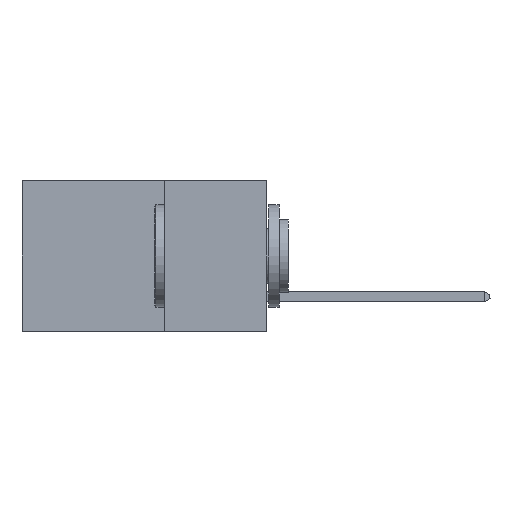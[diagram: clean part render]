
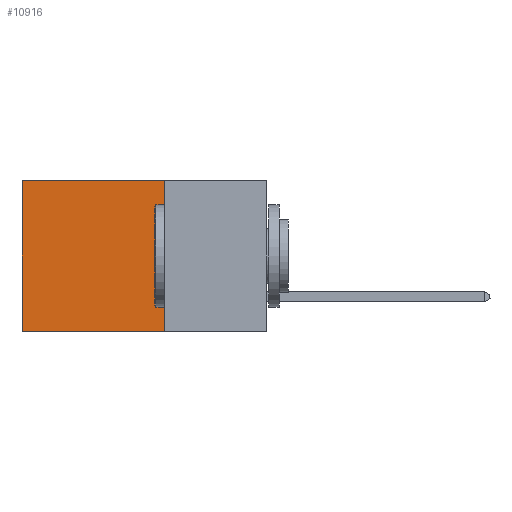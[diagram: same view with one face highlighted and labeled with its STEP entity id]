
A CAD part, left-side view. The second image highlights one B-rep face of the part: STEP entity #10916.
In plain terms, the highlighted planar face has unit normal (-1, 0, 0).
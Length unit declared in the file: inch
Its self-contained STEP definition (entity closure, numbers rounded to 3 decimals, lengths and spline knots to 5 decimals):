
#178 = CARTESIAN_POINT ( 'NONE',  ( 0.2875, 0.25, -0.37 ) ) ;
#617 = CARTESIAN_POINT ( 'NONE',  ( 0.2875, 0.25, 0. ) ) ;
#843 = VERTEX_POINT ( 'NONE', #9537 ) ;
#1072 = VECTOR ( 'NONE', #3567, 39.37008 ) ;
#1185 = DIRECTION ( 'NONE',  ( 0., 1., 0. ) ) ;
#1493 = DIRECTION ( 'NONE',  ( 0., 1., 0. ) ) ;
#1998 = EDGE_CURVE ( 'NONE', #10642, #5314, #9205, .T. ) ;
#2321 = CARTESIAN_POINT ( 'NONE',  ( 0.2875, 0.25, 0. ) ) ;
#2376 = CARTESIAN_POINT ( 'NONE',  ( 0.2875, 0.25, 0. ) ) ;
#2693 = DIRECTION ( 'NONE',  ( 1., 0., 0. ) ) ;
#3020 = VECTOR ( 'NONE', #1185, 39.37008 ) ;
#3567 = DIRECTION ( 'NONE',  ( 0., 0., -1. ) ) ;
#3597 = CARTESIAN_POINT ( 'NONE',  ( 0.2875, 0.6, 0. ) ) ;
#4089 = EDGE_LOOP ( 'NONE', ( #5490, #8207, #4163, #6285 ) ) ;
#4163 = ORIENTED_EDGE ( 'NONE', *, *, #1998, .F. ) ;
#4589 = CARTESIAN_POINT ( 'NONE',  ( 0.2875, 0.25, -0.37 ) ) ;
#5314 = VERTEX_POINT ( 'NONE', #4589 ) ;
#5490 = ORIENTED_EDGE ( 'NONE', *, *, #7692, .T. ) ;
#5806 = LINE ( 'NONE', #178, #3020 ) ;
#6285 = ORIENTED_EDGE ( 'NONE', *, *, #6422, .T. ) ;
#6422 = EDGE_CURVE ( 'NONE', #10642, #9554, #8808, .T. ) ;
#6649 = FACE_OUTER_BOUND ( 'NONE', #4089, .T. ) ;
#7075 = AXIS2_PLACEMENT_3D ( 'NONE', #617, #2693, #9672 ) ;
#7692 = EDGE_CURVE ( 'NONE', #9554, #843, #8828, .T. ) ;
#8000 = EDGE_CURVE ( 'NONE', #5314, #843, #5806, .T. ) ;
#8207 = ORIENTED_EDGE ( 'NONE', *, *, #8000, .F. ) ;
#8420 = DIRECTION ( 'NONE',  ( 0., 0., -1. ) ) ;
#8712 = PLANE ( 'NONE',  #7075 ) ;
#8808 = LINE ( 'NONE', #10462, #9103 ) ;
#8828 = LINE ( 'NONE', #9511, #1072 ) ;
#9103 = VECTOR ( 'NONE', #1493, 39.37008 ) ;
#9205 = LINE ( 'NONE', #2376, #11159 ) ;
#9511 = CARTESIAN_POINT ( 'NONE',  ( 0.2875, 0.6, 0. ) ) ;
#9537 = CARTESIAN_POINT ( 'NONE',  ( 0.2875, 0.6, -0.37 ) ) ;
#9554 = VERTEX_POINT ( 'NONE', #3597 ) ;
#9672 = DIRECTION ( 'NONE',  ( 0., 0., -1. ) ) ;
#10462 = CARTESIAN_POINT ( 'NONE',  ( 0.2875, 0.25, 0. ) ) ;
#10642 = VERTEX_POINT ( 'NONE', #2321 ) ;
#10916 = ADVANCED_FACE ( 'NONE', ( #6649 ), #8712, .F. ) ;
#11159 = VECTOR ( 'NONE', #8420, 39.37008 ) ;
